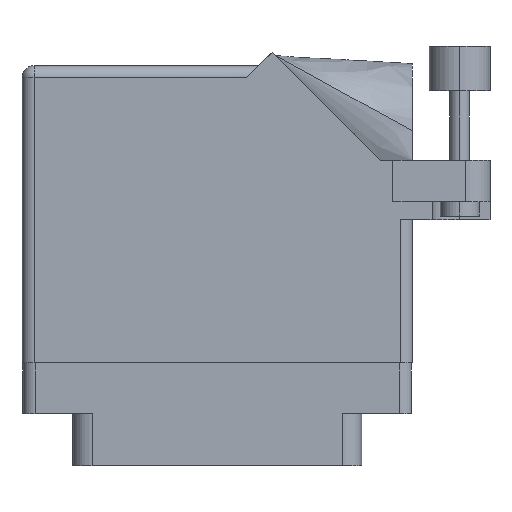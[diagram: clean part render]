
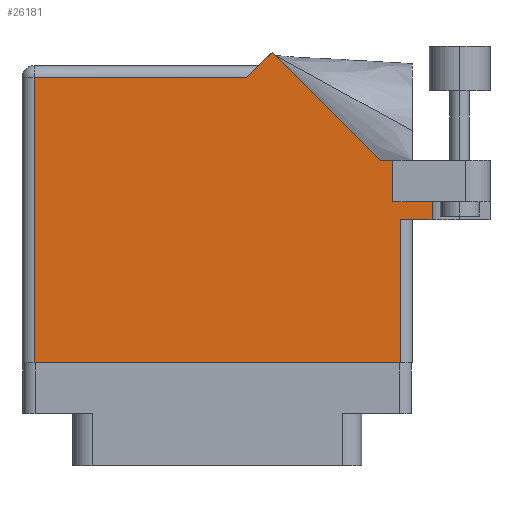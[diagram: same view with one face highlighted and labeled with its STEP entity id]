
A CAD part, front view. The second image highlights one B-rep face of the part: STEP entity #26181.
In plain terms, the highlighted face is planar.
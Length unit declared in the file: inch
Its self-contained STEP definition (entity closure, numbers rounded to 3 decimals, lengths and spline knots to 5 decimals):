
#25 = ORIENTED_EDGE ( 'NONE', *, *, #5199, .T. ) ;
#73 = CARTESIAN_POINT ( 'NONE',  ( 0., 0., 0. ) ) ;
#377 = ORIENTED_EDGE ( 'NONE', *, *, #11042, .T. ) ;
#2018 = LINE ( 'NONE', #28100, #9728 ) ;
#2123 = ORIENTED_EDGE ( 'NONE', *, *, #8951, .T. ) ;
#2532 = EDGE_CURVE ( 'NONE', #2566, #17680, #3139, .T. ) ;
#2566 = VERTEX_POINT ( 'NONE', #14073 ) ;
#2601 = VERTEX_POINT ( 'NONE', #21291 ) ;
#2670 = LINE ( 'NONE', #8544, #29162 ) ;
#2921 = CARTESIAN_POINT ( 'NONE',  ( 1.948, 0.737, 0. ) ) ;
#3139 = LINE ( 'NONE', #24677, #11219 ) ;
#3288 = VERTEX_POINT ( 'NONE', #13270 ) ;
#3704 = ORIENTED_EDGE ( 'NONE', *, *, #22539, .T. ) ;
#4075 = VECTOR ( 'NONE', #6710, 39.37008 ) ;
#4444 = PLANE ( 'NONE',  #7719 ) ;
#4466 = EDGE_CURVE ( 'NONE', #16419, #2601, #9834, .T. ) ;
#4558 = DIRECTION ( 'NONE',  ( -1., 0., 0. ) ) ;
#4902 = DIRECTION ( 'NONE',  ( 0., 0., -1. ) ) ;
#5199 = EDGE_CURVE ( 'NONE', #17680, #23703, #26418, .T. ) ;
#6159 = CARTESIAN_POINT ( 'NONE',  ( 1.28771, 1.60071, 0. ) ) ;
#6447 = VERTEX_POINT ( 'NONE', #32578 ) ;
#6670 = EDGE_CURVE ( 'NONE', #9982, #6447, #23705, .T. ) ;
#6710 = DIRECTION ( 'NONE',  ( -1., 0., 0. ) ) ;
#7063 = VERTEX_POINT ( 'NONE', #18952 ) ;
#7301 = DIRECTION ( 'NONE',  ( 0., -1., 0. ) ) ;
#7719 = AXIS2_PLACEMENT_3D ( 'NONE', #23507, #4902, #4558 ) ;
#7729 = ORIENTED_EDGE ( 'NONE', *, *, #13277, .T. ) ;
#8054 = DIRECTION ( 'NONE',  ( -1., 0., 0. ) ) ;
#8544 = CARTESIAN_POINT ( 'NONE',  ( 1.948, 0.737, 0. ) ) ;
#8951 = EDGE_CURVE ( 'NONE', #7063, #3288, #34474, .T. ) ;
#9140 = DIRECTION ( 'NONE',  ( 0., 1., 0. ) ) ;
#9375 = ORIENTED_EDGE ( 'NONE', *, *, #15602, .F. ) ;
#9728 = VECTOR ( 'NONE', #33181, 39.37008 ) ;
#9834 = LINE ( 'NONE', #33534, #20019 ) ;
#9982 = VERTEX_POINT ( 'NONE', #2921 ) ;
#10106 = EDGE_CURVE ( 'NONE', #3288, #13511, #2018, .T. ) ;
#10215 = CARTESIAN_POINT ( 'NONE',  ( 1.155, 1.468, 0. ) ) ;
#11042 = EDGE_CURVE ( 'NONE', #17848, #2566, #30969, .T. ) ;
#11096 = DIRECTION ( 'NONE',  ( 0., -1., 0. ) ) ;
#11219 = VECTOR ( 'NONE', #11096, 39.37008 ) ;
#11293 = CARTESIAN_POINT ( 'NONE',  ( 1.91, 0.831, 0. ) ) ;
#11595 = ORIENTED_EDGE ( 'NONE', *, *, #4466, .F. ) ;
#11653 = VECTOR ( 'NONE', #9140, 39.37008 ) ;
#13270 = CARTESIAN_POINT ( 'NONE',  ( 1.84442, 1.044, 0. ) ) ;
#13277 = EDGE_CURVE ( 'NONE', #13511, #17848, #34640, .T. ) ;
#13477 = EDGE_CURVE ( 'NONE', #23703, #9982, #2670, .T. ) ;
#13511 = VERTEX_POINT ( 'NONE', #6159 ) ;
#14073 = CARTESIAN_POINT ( 'NONE',  ( 0.062, 1.468, 0. ) ) ;
#14605 = DIRECTION ( 'NONE',  ( 1., 0., 0. ) ) ;
#14948 = LINE ( 'NONE', #28900, #21324 ) ;
#15602 = EDGE_CURVE ( 'NONE', #2601, #6447, #14948, .T. ) ;
#16419 = VERTEX_POINT ( 'NONE', #27965 ) ;
#17385 = FACE_OUTER_BOUND ( 'NONE', #27750, .T. ) ;
#17680 = VERTEX_POINT ( 'NONE', #18170 ) ;
#17843 = ORIENTED_EDGE ( 'NONE', *, *, #6670, .T. ) ;
#17848 = VERTEX_POINT ( 'NONE', #10215 ) ;
#18170 = CARTESIAN_POINT ( 'NONE',  ( 0.062, 0., 0. ) ) ;
#18539 = CARTESIAN_POINT ( 'NONE',  ( 2.41, 1.044, 0. ) ) ;
#18952 = CARTESIAN_POINT ( 'NONE',  ( 1.91, 1.044, 0. ) ) ;
#19128 = VECTOR ( 'NONE', #27035, 39.37008 ) ;
#19318 = ORIENTED_EDGE ( 'NONE', *, *, #10106, .T. ) ;
#19686 = CARTESIAN_POINT ( 'NONE',  ( 2.01, 0.737, 0. ) ) ;
#20019 = VECTOR ( 'NONE', #25585, 39.37008 ) ;
#21127 = VECTOR ( 'NONE', #14605, 39.37008 ) ;
#21291 = CARTESIAN_POINT ( 'NONE',  ( 2.1115, 0.831, 0. ) ) ;
#21324 = VECTOR ( 'NONE', #7301, 39.37008 ) ;
#21987 = CARTESIAN_POINT ( 'NONE',  ( 1.217, 1.53, 0. ) ) ;
#22117 = CARTESIAN_POINT ( 'NONE',  ( 1.948, 0., 0. ) ) ;
#22141 = VECTOR ( 'NONE', #8054, 39.37008 ) ;
#22539 = EDGE_CURVE ( 'NONE', #16419, #7063, #24889, .T. ) ;
#23507 = CARTESIAN_POINT ( 'NONE',  ( 0., 1.53, 0. ) ) ;
#23703 = VERTEX_POINT ( 'NONE', #22117 ) ;
#23705 = LINE ( 'NONE', #19686, #21127 ) ;
#24677 = CARTESIAN_POINT ( 'NONE',  ( 0.062, 0., 0. ) ) ;
#24889 = LINE ( 'NONE', #11293, #11653 ) ;
#25585 = DIRECTION ( 'NONE',  ( 1., 0., 0. ) ) ;
#25784 = ORIENTED_EDGE ( 'NONE', *, *, #13477, .T. ) ;
#26181 = ADVANCED_FACE ( 'NONE', ( #17385 ), #4444, .F. ) ;
#26418 = LINE ( 'NONE', #73, #19128 ) ;
#27035 = DIRECTION ( 'NONE',  ( 1., 0., 0. ) ) ;
#27043 = DIRECTION ( 'NONE',  ( -0.707, -0.707, 0. ) ) ;
#27750 = EDGE_LOOP ( 'NONE', ( #25, #25784, #17843, #9375, #11595, #3704, #2123, #19318, #7729, #377, #30219 ) ) ;
#27965 = CARTESIAN_POINT ( 'NONE',  ( 1.91, 0.831, 0. ) ) ;
#28100 = CARTESIAN_POINT ( 'NONE',  ( 1.84442, 1.044, 0. ) ) ;
#28900 = CARTESIAN_POINT ( 'NONE',  ( 2.1115, 1.16177, 0. ) ) ;
#29162 = VECTOR ( 'NONE', #30373, 39.37008 ) ;
#30219 = ORIENTED_EDGE ( 'NONE', *, *, #2532, .T. ) ;
#30373 = DIRECTION ( 'NONE',  ( 0., 1., 0. ) ) ;
#30430 = VECTOR ( 'NONE', #27043, 39.37008 ) ;
#30969 = LINE ( 'NONE', #31151, #4075 ) ;
#31151 = CARTESIAN_POINT ( 'NONE',  ( 0., 1.468, 0. ) ) ;
#32578 = CARTESIAN_POINT ( 'NONE',  ( 2.1115, 0.737, 0. ) ) ;
#33181 = DIRECTION ( 'NONE',  ( -0.707, 0.707, 0. ) ) ;
#33534 = CARTESIAN_POINT ( 'NONE',  ( 1.91, 0.831, 0. ) ) ;
#34474 = LINE ( 'NONE', #18539, #22141 ) ;
#34640 = LINE ( 'NONE', #21987, #30430 ) ;
